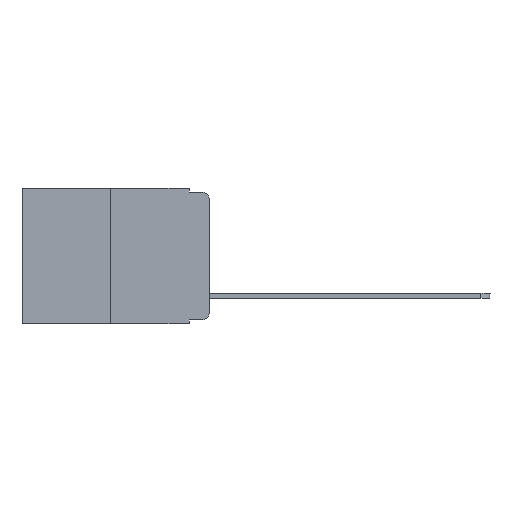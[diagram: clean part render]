
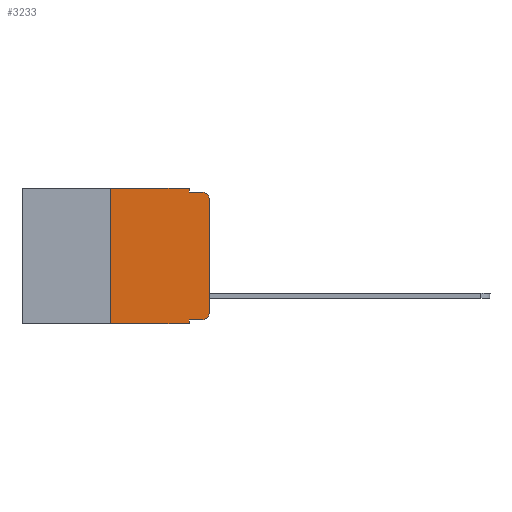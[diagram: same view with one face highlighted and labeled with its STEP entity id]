
A CAD part, left-side view. The second image highlights one B-rep face of the part: STEP entity #3233.
In plain terms, the highlighted planar face has unit normal (-1, 0, 0).
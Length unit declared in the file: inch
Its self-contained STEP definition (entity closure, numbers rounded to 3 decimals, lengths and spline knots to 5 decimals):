
#124 = CARTESIAN_POINT ( 'NONE',  ( 0., 0.473, 0. ) ) ;
#161 = ORIENTED_EDGE ( 'NONE', *, *, #8960, .F. ) ;
#300 = EDGE_CURVE ( 'NONE', #1149, #1350, #9385, .T. ) ;
#304 = DIRECTION ( 'NONE',  ( 0., -1., 0. ) ) ;
#954 = VERTEX_POINT ( 'NONE', #4902 ) ;
#1149 = VERTEX_POINT ( 'NONE', #2790 ) ;
#1350 = VERTEX_POINT ( 'NONE', #5285 ) ;
#1353 = DIRECTION ( 'NONE',  ( 0., 0., -1. ) ) ;
#1403 = VERTEX_POINT ( 'NONE', #2348 ) ;
#1419 = DIRECTION ( 'NONE',  ( 0., -1., 0. ) ) ;
#1527 = ORIENTED_EDGE ( 'NONE', *, *, #2074, .T. ) ;
#1644 = LINE ( 'NONE', #7775, #7807 ) ;
#1652 = DIRECTION ( 'NONE',  ( 0., 0., -1. ) ) ;
#1863 = CARTESIAN_POINT ( 'NONE',  ( 0., 0.051, 0. ) ) ;
#1910 = CARTESIAN_POINT ( 'NONE',  ( 0., 0., -0.313 ) ) ;
#1915 = CIRCLE ( 'NONE', #7980, 0.02 ) ;
#1950 = EDGE_CURVE ( 'NONE', #954, #7222, #2281, .T. ) ;
#2074 = EDGE_CURVE ( 'NONE', #9304, #7169, #5777, .T. ) ;
#2219 = FACE_OUTER_BOUND ( 'NONE', #2926, .T. ) ;
#2281 = LINE ( 'NONE', #6229, #5885 ) ;
#2348 = CARTESIAN_POINT ( 'NONE',  ( 0., 0.051, -0.343 ) ) ;
#2358 = CARTESIAN_POINT ( 'NONE',  ( 0., 0.051, -0.01 ) ) ;
#2496 = DIRECTION ( 'NONE',  ( 0., 0., 1. ) ) ;
#2507 = DIRECTION ( 'NONE',  ( -1., 0., 0. ) ) ;
#2587 = EDGE_CURVE ( 'NONE', #7222, #7851, #8411, .T. ) ;
#2682 = VERTEX_POINT ( 'NONE', #2358 ) ;
#2790 = CARTESIAN_POINT ( 'NONE',  ( 0., 0.051, -0.333 ) ) ;
#2851 = EDGE_CURVE ( 'NONE', #2682, #7169, #5124, .T. ) ;
#2926 = EDGE_LOOP ( 'NONE', ( #9025, #1527, #6957, #161, #7621, #5607, #3401, #9049, #6204, #7319 ) ) ;
#3016 = AXIS2_PLACEMENT_3D ( 'NONE', #9442, #5718, #7244 ) ;
#3233 = ADVANCED_FACE ( 'NONE', ( #2219 ), #8492, .F. ) ;
#3289 = CARTESIAN_POINT ( 'NONE',  ( 0., 0.02, -0.01 ) ) ;
#3300 = DIRECTION ( 'NONE',  ( 0., 0., 1. ) ) ;
#3401 = ORIENTED_EDGE ( 'NONE', *, *, #8928, .T. ) ;
#3435 = AXIS2_PLACEMENT_3D ( 'NONE', #8425, #8563, #9164 ) ;
#3937 = VECTOR ( 'NONE', #8110, 39.37008 ) ;
#4902 = CARTESIAN_POINT ( 'NONE',  ( 0., 0.25, -0.343 ) ) ;
#4995 = VECTOR ( 'NONE', #1353, 39.37008 ) ;
#5124 = LINE ( 'NONE', #6435, #6183 ) ;
#5285 = CARTESIAN_POINT ( 'NONE',  ( 0., 0.02, -0.333 ) ) ;
#5598 = DIRECTION ( 'NONE',  ( 0., -1., 0. ) ) ;
#5607 = ORIENTED_EDGE ( 'NONE', *, *, #1950, .F. ) ;
#5635 = CARTESIAN_POINT ( 'NONE',  ( 0., 0.051, 0. ) ) ;
#5706 = LINE ( 'NONE', #5817, #4995 ) ;
#5718 = DIRECTION ( 'NONE',  ( -1., 0., 0. ) ) ;
#5777 = CIRCLE ( 'NONE', #3016, 0.02 ) ;
#5817 = CARTESIAN_POINT ( 'NONE',  ( 0., 0.051, 0. ) ) ;
#5885 = VECTOR ( 'NONE', #3300, 39.37008 ) ;
#6134 = VERTEX_POINT ( 'NONE', #1910 ) ;
#6183 = VECTOR ( 'NONE', #5598, 39.37008 ) ;
#6204 = ORIENTED_EDGE ( 'NONE', *, *, #300, .T. ) ;
#6229 = CARTESIAN_POINT ( 'NONE',  ( 0., 0.25, 0. ) ) ;
#6247 = CARTESIAN_POINT ( 'NONE',  ( 0., 0.25, 0. ) ) ;
#6435 = CARTESIAN_POINT ( 'NONE',  ( 0., 0.051, -0.01 ) ) ;
#6555 = LINE ( 'NONE', #5635, #7560 ) ;
#6714 = VECTOR ( 'NONE', #1419, 39.37008 ) ;
#6740 = EDGE_CURVE ( 'NONE', #1149, #1403, #5706, .T. ) ;
#6933 = VECTOR ( 'NONE', #2496, 39.37008 ) ;
#6957 = ORIENTED_EDGE ( 'NONE', *, *, #2851, .F. ) ;
#6972 = CARTESIAN_POINT ( 'NONE',  ( 0., 0.02, -0.313 ) ) ;
#7169 = VERTEX_POINT ( 'NONE', #3289 ) ;
#7222 = VERTEX_POINT ( 'NONE', #6247 ) ;
#7244 = DIRECTION ( 'NONE',  ( 0., 0., -1. ) ) ;
#7319 = ORIENTED_EDGE ( 'NONE', *, *, #9310, .T. ) ;
#7560 = VECTOR ( 'NONE', #8536, 39.37008 ) ;
#7581 = CARTESIAN_POINT ( 'NONE',  ( 0., 0., -0.03 ) ) ;
#7621 = ORIENTED_EDGE ( 'NONE', *, *, #2587, .F. ) ;
#7645 = CARTESIAN_POINT ( 'NONE',  ( 0., 0., 0. ) ) ;
#7775 = CARTESIAN_POINT ( 'NONE',  ( 0., 0.473, -0.343 ) ) ;
#7807 = VECTOR ( 'NONE', #304, 39.37008 ) ;
#7851 = VERTEX_POINT ( 'NONE', #1863 ) ;
#7980 = AXIS2_PLACEMENT_3D ( 'NONE', #6972, #2507, #1652 ) ;
#8110 = DIRECTION ( 'NONE',  ( 0., -1., 0. ) ) ;
#8411 = LINE ( 'NONE', #124, #6714 ) ;
#8425 = CARTESIAN_POINT ( 'NONE',  ( 0., 0.473, 0. ) ) ;
#8492 = PLANE ( 'NONE',  #3435 ) ;
#8536 = DIRECTION ( 'NONE',  ( 0., 0., -1. ) ) ;
#8563 = DIRECTION ( 'NONE',  ( 1., 0., 0. ) ) ;
#8928 = EDGE_CURVE ( 'NONE', #954, #1403, #1644, .T. ) ;
#8960 = EDGE_CURVE ( 'NONE', #7851, #2682, #6555, .T. ) ;
#9025 = ORIENTED_EDGE ( 'NONE', *, *, #9148, .T. ) ;
#9049 = ORIENTED_EDGE ( 'NONE', *, *, #6740, .F. ) ;
#9148 = EDGE_CURVE ( 'NONE', #6134, #9304, #9332, .T. ) ;
#9164 = DIRECTION ( 'NONE',  ( 0., 0., -1. ) ) ;
#9304 = VERTEX_POINT ( 'NONE', #7581 ) ;
#9310 = EDGE_CURVE ( 'NONE', #1350, #6134, #1915, .T. ) ;
#9332 = LINE ( 'NONE', #7645, #6933 ) ;
#9385 = LINE ( 'NONE', #9528, #3937 ) ;
#9442 = CARTESIAN_POINT ( 'NONE',  ( 0., 0.02, -0.03 ) ) ;
#9528 = CARTESIAN_POINT ( 'NONE',  ( 0., 0.051, -0.333 ) ) ;
